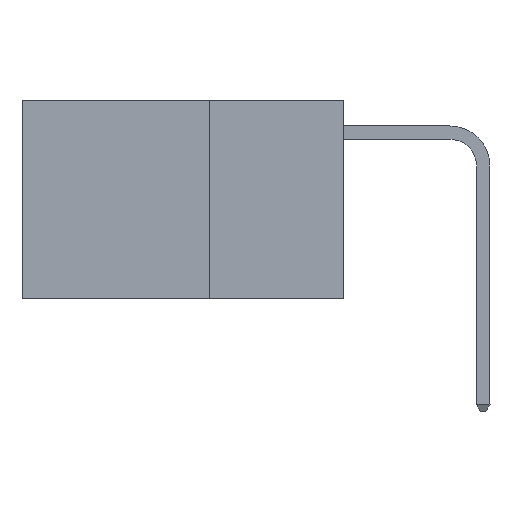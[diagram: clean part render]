
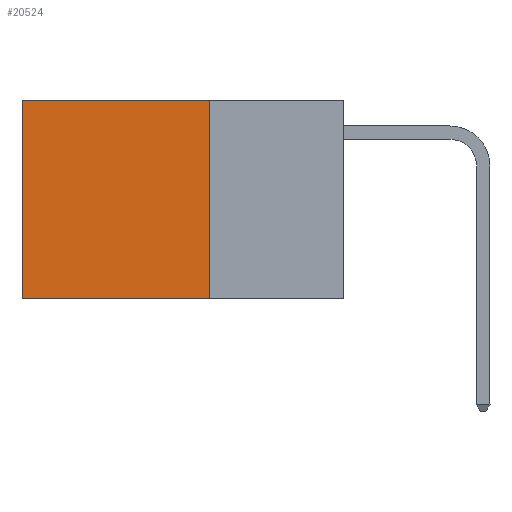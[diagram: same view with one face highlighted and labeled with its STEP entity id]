
A CAD part, left-side view. The second image highlights one B-rep face of the part: STEP entity #20524.
In plain terms, the highlighted planar face has unit normal (-1, 0, 0).
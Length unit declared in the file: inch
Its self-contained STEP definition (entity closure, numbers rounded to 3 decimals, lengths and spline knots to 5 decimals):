
#457 = ORIENTED_EDGE ( 'NONE', *, *, #1709, .F. ) ;
#1251 = VECTOR ( 'NONE', #4418, 39.37008 ) ;
#1709 = EDGE_CURVE ( 'NONE', #5168, #5081, #20537, .T. ) ;
#4376 = CARTESIAN_POINT ( 'NONE',  ( 0.2625, 0.25, -0.37 ) ) ;
#4418 = DIRECTION ( 'NONE',  ( 0., 1., 0. ) ) ;
#4490 = CARTESIAN_POINT ( 'NONE',  ( 0.2625, 0.25, 0. ) ) ;
#4830 = CARTESIAN_POINT ( 'NONE',  ( 0.2625, 0.6, -0.37 ) ) ;
#4997 = DIRECTION ( 'NONE',  ( 0., 0., -1. ) ) ;
#5080 = DIRECTION ( 'NONE',  ( 0., 0., -1. ) ) ;
#5081 = VERTEX_POINT ( 'NONE', #10010 ) ;
#5168 = VERTEX_POINT ( 'NONE', #8336 ) ;
#5766 = VECTOR ( 'NONE', #5080, 39.37008 ) ;
#7678 = CARTESIAN_POINT ( 'NONE',  ( 0.2625, 0.6, 0. ) ) ;
#7950 = VERTEX_POINT ( 'NONE', #4830 ) ;
#7993 = VECTOR ( 'NONE', #4997, 39.37008 ) ;
#8028 = EDGE_CURVE ( 'NONE', #14365, #7950, #17857, .T. ) ;
#8336 = CARTESIAN_POINT ( 'NONE',  ( 0.2625, 0.25, 0. ) ) ;
#8802 = CARTESIAN_POINT ( 'NONE',  ( 0.2625, 0.6, 0. ) ) ;
#9120 = DIRECTION ( 'NONE',  ( 1., 0., 0. ) ) ;
#9320 = ORIENTED_EDGE ( 'NONE', *, *, #11440, .T. ) ;
#9977 = VECTOR ( 'NONE', #10087, 39.37008 ) ;
#10010 = CARTESIAN_POINT ( 'NONE',  ( 0.2625, 0.25, -0.37 ) ) ;
#10087 = DIRECTION ( 'NONE',  ( 0., 1., 0. ) ) ;
#10506 = EDGE_LOOP ( 'NONE', ( #23163, #23149, #457, #9320 ) ) ;
#11440 = EDGE_CURVE ( 'NONE', #5168, #14365, #21075, .T. ) ;
#12676 = FACE_OUTER_BOUND ( 'NONE', #10506, .T. ) ;
#13317 = EDGE_CURVE ( 'NONE', #5081, #7950, #19793, .T. ) ;
#14365 = VERTEX_POINT ( 'NONE', #7678 ) ;
#14670 = PLANE ( 'NONE',  #20338 ) ;
#17451 = CARTESIAN_POINT ( 'NONE',  ( 0.2625, 0.25, 0. ) ) ;
#17857 = LINE ( 'NONE', #8802, #7993 ) ;
#19793 = LINE ( 'NONE', #4376, #9977 ) ;
#20166 = CARTESIAN_POINT ( 'NONE',  ( 0.2625, 0.25, 0. ) ) ;
#20338 = AXIS2_PLACEMENT_3D ( 'NONE', #20166, #9120, #21959 ) ;
#20524 = ADVANCED_FACE ( 'NONE', ( #12676 ), #14670, .F. ) ;
#20537 = LINE ( 'NONE', #4490, #5766 ) ;
#21075 = LINE ( 'NONE', #17451, #1251 ) ;
#21959 = DIRECTION ( 'NONE',  ( 0., 0., -1. ) ) ;
#23149 = ORIENTED_EDGE ( 'NONE', *, *, #13317, .F. ) ;
#23163 = ORIENTED_EDGE ( 'NONE', *, *, #8028, .T. ) ;
